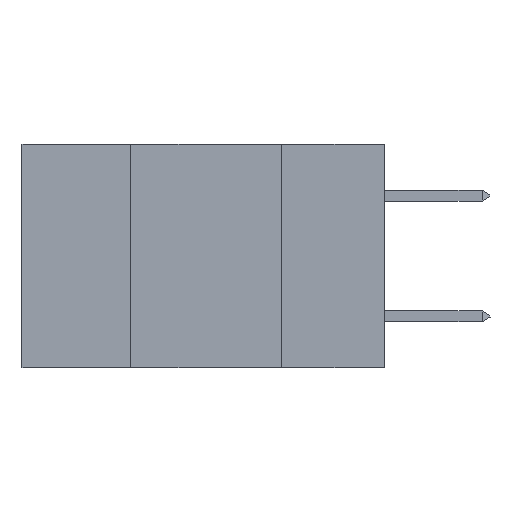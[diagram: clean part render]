
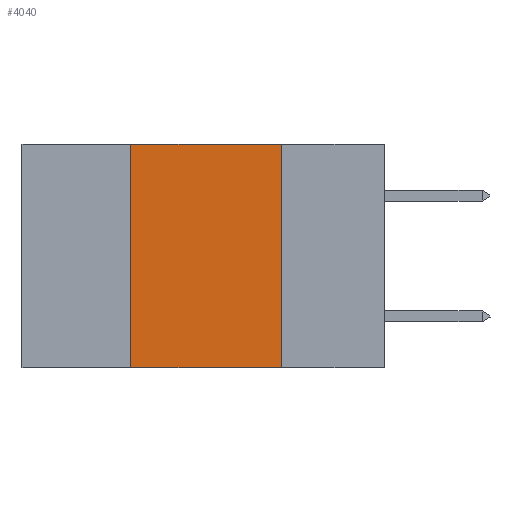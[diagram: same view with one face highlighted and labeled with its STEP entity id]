
A CAD part, left-side view. The second image highlights one B-rep face of the part: STEP entity #4040.
In plain terms, the highlighted planar face has unit normal (-1, 0, 0).
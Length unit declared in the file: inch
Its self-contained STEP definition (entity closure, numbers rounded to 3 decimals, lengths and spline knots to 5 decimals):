
#247 = EDGE_CURVE ( 'NONE', #8682, #8033, #5541, .T. ) ;
#299 = ORIENTED_EDGE ( 'NONE', *, *, #5788, .F. ) ;
#559 = LINE ( 'NONE', #8211, #5795 ) ;
#829 = ORIENTED_EDGE ( 'NONE', *, *, #247, .F. ) ;
#1033 = DIRECTION ( 'NONE',  ( 0., 0., 1. ) ) ;
#1401 = LINE ( 'NONE', #5887, #9643 ) ;
#2119 = EDGE_LOOP ( 'NONE', ( #2525, #829, #299, #4322 ) ) ;
#2525 = ORIENTED_EDGE ( 'NONE', *, *, #2527, .F. ) ;
#2527 = EDGE_CURVE ( 'NONE', #8033, #5961, #1401, .T. ) ;
#2974 = CARTESIAN_POINT ( 'NONE',  ( 0., 0.17, -0.37 ) ) ;
#3050 = CARTESIAN_POINT ( 'NONE',  ( 0., 0.42, 0. ) ) ;
#3417 = VECTOR ( 'NONE', #1033, 39.37008 ) ;
#3741 = AXIS2_PLACEMENT_3D ( 'NONE', #3904, #9504, #9470 ) ;
#3904 = CARTESIAN_POINT ( 'NONE',  ( 0., 0.6, 0. ) ) ;
#4040 = ADVANCED_FACE ( 'NONE', ( #6591 ), #7046, .F. ) ;
#4303 = DIRECTION ( 'NONE',  ( 0., 0., -1. ) ) ;
#4322 = ORIENTED_EDGE ( 'NONE', *, *, #9848, .T. ) ;
#4761 = CARTESIAN_POINT ( 'NONE',  ( 0., 0.6, 0. ) ) ;
#4780 = LINE ( 'NONE', #9109, #3417 ) ;
#5541 = LINE ( 'NONE', #4761, #8056 ) ;
#5788 = EDGE_CURVE ( 'NONE', #9519, #8682, #4780, .T. ) ;
#5795 = VECTOR ( 'NONE', #8278, 39.37008 ) ;
#5887 = CARTESIAN_POINT ( 'NONE',  ( 0., 0.17, 0. ) ) ;
#5961 = VERTEX_POINT ( 'NONE', #2974 ) ;
#6591 = FACE_OUTER_BOUND ( 'NONE', #2119, .T. ) ;
#7046 = PLANE ( 'NONE',  #3741 ) ;
#7544 = CARTESIAN_POINT ( 'NONE',  ( 0., 0.17, 0. ) ) ;
#7809 = DIRECTION ( 'NONE',  ( 0., -1., 0. ) ) ;
#8033 = VERTEX_POINT ( 'NONE', #7544 ) ;
#8056 = VECTOR ( 'NONE', #7809, 39.37008 ) ;
#8211 = CARTESIAN_POINT ( 'NONE',  ( 0., 0.6, -0.37 ) ) ;
#8278 = DIRECTION ( 'NONE',  ( 0., -1., 0. ) ) ;
#8682 = VERTEX_POINT ( 'NONE', #3050 ) ;
#8809 = CARTESIAN_POINT ( 'NONE',  ( 0., 0.42, -0.37 ) ) ;
#9109 = CARTESIAN_POINT ( 'NONE',  ( 0., 0.42, 0. ) ) ;
#9470 = DIRECTION ( 'NONE',  ( 0., 0., -1. ) ) ;
#9504 = DIRECTION ( 'NONE',  ( 1., 0., 0. ) ) ;
#9519 = VERTEX_POINT ( 'NONE', #8809 ) ;
#9643 = VECTOR ( 'NONE', #4303, 39.37008 ) ;
#9848 = EDGE_CURVE ( 'NONE', #9519, #5961, #559, .T. ) ;
